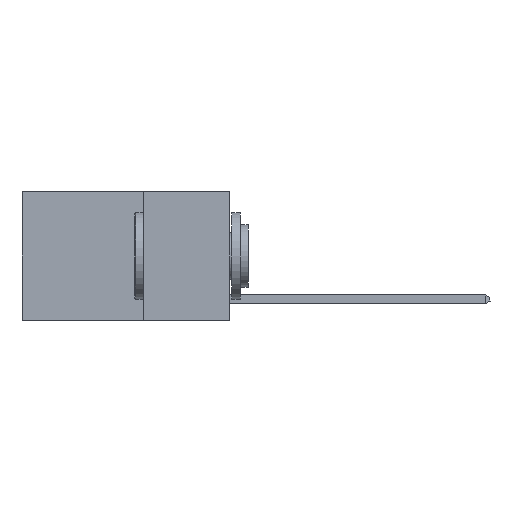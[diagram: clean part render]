
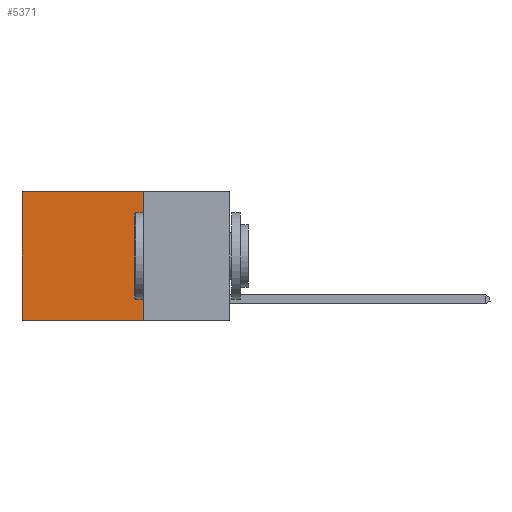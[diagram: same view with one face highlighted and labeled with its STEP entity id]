
A CAD part, left-side view. The second image highlights one B-rep face of the part: STEP entity #5371.
In plain terms, the highlighted planar face has unit normal (-1, 0, 0).
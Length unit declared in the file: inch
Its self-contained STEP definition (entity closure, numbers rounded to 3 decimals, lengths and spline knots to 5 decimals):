
#84 = CARTESIAN_POINT ( 'NONE',  ( 0.2625, 0.25, -0.37 ) ) ;
#487 = VERTEX_POINT ( 'NONE', #14514 ) ;
#835 = CARTESIAN_POINT ( 'NONE',  ( 0.2625, 0.25, 0. ) ) ;
#2631 = EDGE_CURVE ( 'NONE', #14712, #18727, #5390, .T. ) ;
#2662 = VERTEX_POINT ( 'NONE', #14691 ) ;
#4039 = LINE ( 'NONE', #9371, #16220 ) ;
#4370 = CARTESIAN_POINT ( 'NONE',  ( 0.2625, 0.25, 0. ) ) ;
#5371 = ADVANCED_FACE ( 'NONE', ( #17829 ), #13544, .F. ) ;
#5390 = LINE ( 'NONE', #9989, #17074 ) ;
#5907 = DIRECTION ( 'NONE',  ( 1., 0., 0. ) ) ;
#6122 = VECTOR ( 'NONE', #9836, 39.37008 ) ;
#6738 = CARTESIAN_POINT ( 'NONE',  ( 0.2625, 0.6, 0. ) ) ;
#7080 = AXIS2_PLACEMENT_3D ( 'NONE', #4370, #5907, #16577 ) ;
#7348 = ORIENTED_EDGE ( 'NONE', *, *, #9756, .F. ) ;
#7880 = ORIENTED_EDGE ( 'NONE', *, *, #2631, .T. ) ;
#9371 = CARTESIAN_POINT ( 'NONE',  ( 0.2625, 0.25, 0. ) ) ;
#9392 = DIRECTION ( 'NONE',  ( 0., 1., 0. ) ) ;
#9484 = ORIENTED_EDGE ( 'NONE', *, *, #14155, .F. ) ;
#9756 = EDGE_CURVE ( 'NONE', #487, #2662, #18614, .T. ) ;
#9836 = DIRECTION ( 'NONE',  ( 0., 0., -1. ) ) ;
#9989 = CARTESIAN_POINT ( 'NONE',  ( 0.2625, 0.25, 0. ) ) ;
#10010 = VECTOR ( 'NONE', #9392, 39.37008 ) ;
#10484 = EDGE_CURVE ( 'NONE', #18727, #2662, #11119, .T. ) ;
#10925 = DIRECTION ( 'NONE',  ( 0., 0., -1. ) ) ;
#11119 = LINE ( 'NONE', #6738, #6122 ) ;
#13544 = PLANE ( 'NONE',  #7080 ) ;
#14155 = EDGE_CURVE ( 'NONE', #14712, #487, #4039, .T. ) ;
#14504 = ORIENTED_EDGE ( 'NONE', *, *, #10484, .T. ) ;
#14514 = CARTESIAN_POINT ( 'NONE',  ( 0.2625, 0.25, -0.37 ) ) ;
#14691 = CARTESIAN_POINT ( 'NONE',  ( 0.2625, 0.6, -0.37 ) ) ;
#14692 = EDGE_LOOP ( 'NONE', ( #14504, #7348, #9484, #7880 ) ) ;
#14712 = VERTEX_POINT ( 'NONE', #835 ) ;
#16220 = VECTOR ( 'NONE', #10925, 39.37008 ) ;
#16577 = DIRECTION ( 'NONE',  ( 0., 0., -1. ) ) ;
#16897 = CARTESIAN_POINT ( 'NONE',  ( 0.2625, 0.6, 0. ) ) ;
#17074 = VECTOR ( 'NONE', #17669, 39.37008 ) ;
#17669 = DIRECTION ( 'NONE',  ( 0., 1., 0. ) ) ;
#17829 = FACE_OUTER_BOUND ( 'NONE', #14692, .T. ) ;
#18614 = LINE ( 'NONE', #84, #10010 ) ;
#18727 = VERTEX_POINT ( 'NONE', #16897 ) ;
